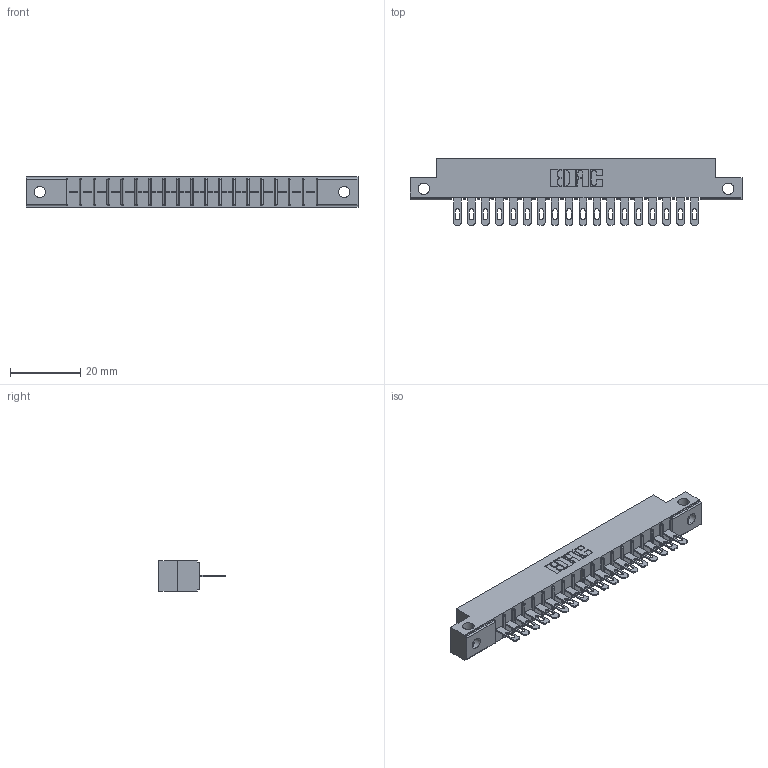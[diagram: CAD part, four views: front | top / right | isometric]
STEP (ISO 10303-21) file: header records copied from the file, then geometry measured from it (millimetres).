
FILE_DESCRIPTION (( 'STEP AP203' ), '1' );
FILE_NAME ('316-018-500-112.STEP', '2020-09-20T20:44:26', ( '' ), ( '' ), 'SwSTEP 2.0', 'SolidWorks 2020', '' );
FILE_SCHEMA (( 'CONFIG_CONTROL_DESIGN' ));
Length unit declared in the file: inch
Products named in the file (3): 306-290-001_100; 316-018-500-112; 306 Part_.128 Dia
Assembly tree (19 placements, depth 2):
  316-018-500-112
    306 Part_.128 Dia
    306-290-001_100  x18
Bounding box: 94.34 x 18.87 x 8.71 mm (x, y, z)
Volume: 6360.5 mm3; surface area: 9500.1 mm2
Topology: 19 solids, 19 shells, 1496 faces, 4222 edges, 2712 vertices
Faces by surface type: plane 968, cylinder 456, sphere 72
Entity records: 20465 total; most frequent: CARTESIAN_POINT 3481, ORIENTED_EDGE 3404, DIRECTION 3374, EDGE_CURVE 1702, LINE 1300, VECTOR 1300, VERTEX_POINT 1080, AXIS2_PLACEMENT_3D 1037
